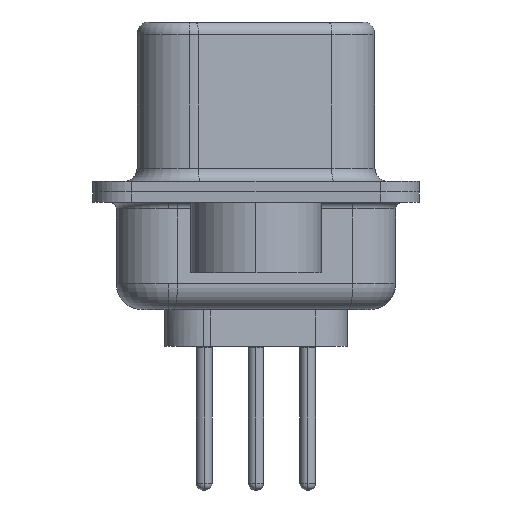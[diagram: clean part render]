
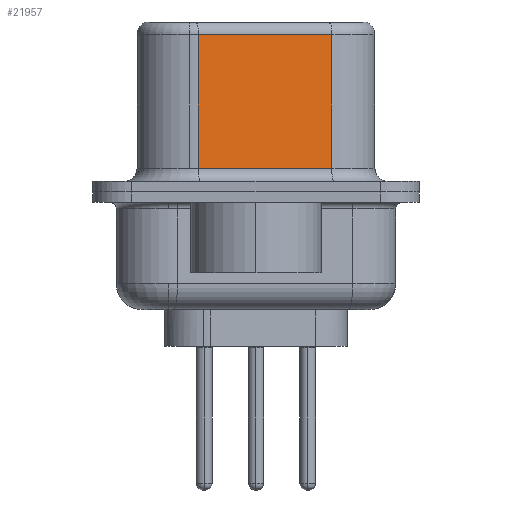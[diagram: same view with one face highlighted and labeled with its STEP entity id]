
A CAD part, left-side view. The second image highlights one B-rep face of the part: STEP entity #21957.
In plain terms, the highlighted planar face has unit normal (-0.985, -0.174, 0).
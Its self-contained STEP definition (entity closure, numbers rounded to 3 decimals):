
#110 = EDGE_CURVE ( 'NONE', #7281, #14574, #11621, .T. ) ;
#1104 = DIRECTION ( 'NONE',  ( -0.174, 0.985, 0. ) ) ;
#1463 = DIRECTION ( 'NONE',  ( 0.174, -0.985, 0. ) ) ;
#1507 = DIRECTION ( 'NONE',  ( -0.174, 0.985, 0. ) ) ;
#2627 = EDGE_LOOP ( 'NONE', ( #25352, #4954, #16177, #10441 ) ) ;
#3184 = DIRECTION ( 'NONE',  ( 0., 0., -1. ) ) ;
#3603 = CARTESIAN_POINT ( 'NONE',  ( 4.58, -2.897, 0.9 ) ) ;
#4883 = CARTESIAN_POINT ( 'NONE',  ( 3.68, 2.203, 6.52 ) ) ;
#4954 = ORIENTED_EDGE ( 'NONE', *, *, #21497, .T. ) ;
#5165 = DIRECTION ( 'NONE',  ( 0., 0., -1. ) ) ;
#5707 = EDGE_CURVE ( 'NONE', #11391, #7281, #17449, .T. ) ;
#6119 = VECTOR ( 'NONE', #1463, 1000. ) ;
#6224 = CARTESIAN_POINT ( 'NONE',  ( 4.58, -2.897, 6.02 ) ) ;
#7281 = VERTEX_POINT ( 'NONE', #23268 ) ;
#7300 = PLANE ( 'NONE',  #11592 ) ;
#7496 = CARTESIAN_POINT ( 'NONE',  ( 3.68, 2.203, 6.02 ) ) ;
#7802 = FACE_OUTER_BOUND ( 'NONE', #2627, .T. ) ;
#9393 = CARTESIAN_POINT ( 'NONE',  ( 4.58, -2.897, 6.52 ) ) ;
#10441 = ORIENTED_EDGE ( 'NONE', *, *, #110, .T. ) ;
#11391 = VERTEX_POINT ( 'NONE', #7496 ) ;
#11592 = AXIS2_PLACEMENT_3D ( 'NONE', #9393, #13541, #1104 ) ;
#11621 = LINE ( 'NONE', #25342, #6119 ) ;
#13384 = CARTESIAN_POINT ( 'NONE',  ( 4.58, -2.897, 6.52 ) ) ;
#13541 = DIRECTION ( 'NONE',  ( 0.985, 0.174, 0. ) ) ;
#14574 = VERTEX_POINT ( 'NONE', #3603 ) ;
#15536 = VERTEX_POINT ( 'NONE', #6224 ) ;
#16177 = ORIENTED_EDGE ( 'NONE', *, *, #5707, .T. ) ;
#16508 = VECTOR ( 'NONE', #5165, 1000. ) ;
#17449 = LINE ( 'NONE', #4883, #22217 ) ;
#18090 = VECTOR ( 'NONE', #1507, 1000. ) ;
#18705 = LINE ( 'NONE', #26052, #18090 ) ;
#21330 = EDGE_CURVE ( 'NONE', #15536, #14574, #21906, .T. ) ;
#21497 = EDGE_CURVE ( 'NONE', #15536, #11391, #18705, .T. ) ;
#21906 = LINE ( 'NONE', #13384, #16508 ) ;
#21957 = ADVANCED_FACE ( 'NONE', ( #7802 ), #7300, .F. ) ;
#22217 = VECTOR ( 'NONE', #3184, 1000. ) ;
#23268 = CARTESIAN_POINT ( 'NONE',  ( 3.68, 2.203, 0.9 ) ) ;
#25342 = CARTESIAN_POINT ( 'NONE',  ( 4.58, -2.897, 0.9 ) ) ;
#25352 = ORIENTED_EDGE ( 'NONE', *, *, #21330, .F. ) ;
#26052 = CARTESIAN_POINT ( 'NONE',  ( 4.58, -2.897, 6.02 ) ) ;
